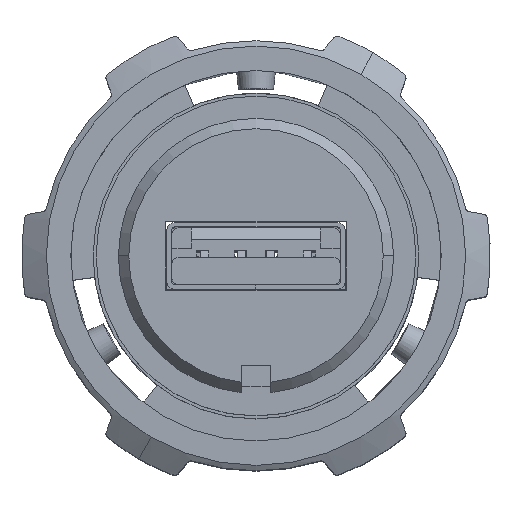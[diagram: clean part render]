
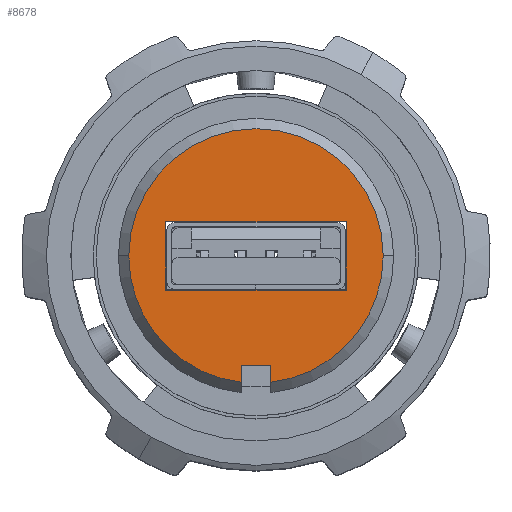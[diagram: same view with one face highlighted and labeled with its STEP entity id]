
A CAD part, top view. The second image highlights one B-rep face of the part: STEP entity #8678.
In plain terms, the highlighted face is planar.
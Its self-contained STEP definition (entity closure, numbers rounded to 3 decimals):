
#571 = ORIENTED_EDGE ( 'NONE', *, *, #32769, .F. ) ;
#1114 = VECTOR ( 'NONE', #8044, 1000. ) ;
#1284 = VERTEX_POINT ( 'NONE', #28945 ) ;
#1845 = ORIENTED_EDGE ( 'NONE', *, *, #14974, .F. ) ;
#2057 = DIRECTION ( 'NONE',  ( 0., 0., -1. ) ) ;
#2321 = LINE ( 'NONE', #23483, #1114 ) ;
#2483 = CIRCLE ( 'NONE', #13018, 8.55 ) ;
#3827 = EDGE_CURVE ( 'NONE', #29091, #33303, #2321, .T. ) ;
#4218 = DIRECTION ( 'NONE',  ( 0., -1., 0. ) ) ;
#4243 = ORIENTED_EDGE ( 'NONE', *, *, #15175, .F. ) ;
#4563 = LINE ( 'NONE', #15160, #25187 ) ;
#5226 = DIRECTION ( 'NONE',  ( 0., 0., -1. ) ) ;
#5228 = VERTEX_POINT ( 'NONE', #34061 ) ;
#5589 = VERTEX_POINT ( 'NONE', #20639 ) ;
#6197 = LINE ( 'NONE', #6367, #14381 ) ;
#6367 = CARTESIAN_POINT ( 'NONE',  ( -27.9, -2.3, 0. ) ) ;
#6452 = LINE ( 'NONE', #23599, #9389 ) ;
#6960 = VERTEX_POINT ( 'NONE', #18291 ) ;
#7272 = EDGE_LOOP ( 'NONE', ( #11603, #23255, #19505, #8201 ) ) ;
#7337 = FACE_OUTER_BOUND ( 'NONE', #19767, .T. ) ;
#7971 = AXIS2_PLACEMENT_3D ( 'NONE', #21669, #32272, #32097 ) ;
#8044 = DIRECTION ( 'NONE',  ( 0., -1., 0. ) ) ;
#8084 = VERTEX_POINT ( 'NONE', #21839 ) ;
#8201 = ORIENTED_EDGE ( 'NONE', *, *, #18964, .F. ) ;
#8480 = CARTESIAN_POINT ( 'NONE',  ( -27.9, -2.3, 6.05 ) ) ;
#8678 = ADVANCED_FACE ( 'NONE', ( #20852, #7337 ), #28850, .F. ) ;
#9386 = VECTOR ( 'NONE', #15297, 1000. ) ;
#9389 = VECTOR ( 'NONE', #17720, 1000. ) ;
#9442 = CARTESIAN_POINT ( 'NONE',  ( -27.9, 0., 8.55 ) ) ;
#9925 = LINE ( 'NONE', #15817, #9386 ) ;
#11046 = VECTOR ( 'NONE', #2057, 1000. ) ;
#11603 = ORIENTED_EDGE ( 'NONE', *, *, #29105, .F. ) ;
#12642 = CARTESIAN_POINT ( 'NONE',  ( -27.9, 2.3, 0. ) ) ;
#12925 = CIRCLE ( 'NONE', #32345, 8.55 ) ;
#13018 = AXIS2_PLACEMENT_3D ( 'NONE', #28632, #20814, #15802 ) ;
#14381 = VECTOR ( 'NONE', #32923, 1000. ) ;
#14974 = EDGE_CURVE ( 'NONE', #1284, #33925, #12925, .T. ) ;
#15160 = CARTESIAN_POINT ( 'NONE',  ( -27.9, 0., -1. ) ) ;
#15175 = EDGE_CURVE ( 'NONE', #5589, #1284, #26248, .T. ) ;
#15255 = LINE ( 'NONE', #12642, #11046 ) ;
#15297 = DIRECTION ( 'NONE',  ( 0., 1., 0. ) ) ;
#15527 = CARTESIAN_POINT ( 'NONE',  ( -27.9, -7.396, -1. ) ) ;
#15802 = DIRECTION ( 'NONE',  ( 0., 0., -1. ) ) ;
#15817 = CARTESIAN_POINT ( 'NONE',  ( -27.9, 0., 1. ) ) ;
#17163 = VECTOR ( 'NONE', #5226, 1000. ) ;
#17720 = DIRECTION ( 'NONE',  ( 0., 1., 0. ) ) ;
#17922 = DIRECTION ( 'NONE',  ( 0., 0., -1. ) ) ;
#18291 = CARTESIAN_POINT ( 'NONE',  ( -27.9, -8.491, 1. ) ) ;
#18566 = EDGE_CURVE ( 'NONE', #6960, #5228, #9925, .T. ) ;
#18964 = EDGE_CURVE ( 'NONE', #8084, #29091, #15255, .T. ) ;
#19505 = ORIENTED_EDGE ( 'NONE', *, *, #3827, .F. ) ;
#19623 = CARTESIAN_POINT ( 'NONE',  ( -27.9, 2.3, -6.05 ) ) ;
#19640 = CARTESIAN_POINT ( 'NONE',  ( -27.9, 0., 0. ) ) ;
#19767 = EDGE_LOOP ( 'NONE', ( #32640, #29613, #1845, #4243, #571, #33264 ) ) ;
#20324 = LINE ( 'NONE', #23262, #17163 ) ;
#20639 = CARTESIAN_POINT ( 'NONE',  ( -27.9, -8.491, -1. ) ) ;
#20650 = CARTESIAN_POINT ( 'NONE',  ( -27.9, -2.3, -6.05 ) ) ;
#20814 = DIRECTION ( 'NONE',  ( 1., 0., 0. ) ) ;
#20852 = FACE_BOUND ( 'NONE', #7272, .T. ) ;
#21669 = CARTESIAN_POINT ( 'NONE',  ( -27.9, 0., 0. ) ) ;
#21839 = CARTESIAN_POINT ( 'NONE',  ( -27.9, 2.3, 6.05 ) ) ;
#22414 = DIRECTION ( 'NONE',  ( 1., 0., 0. ) ) ;
#22799 = VERTEX_POINT ( 'NONE', #15527 ) ;
#23255 = ORIENTED_EDGE ( 'NONE', *, *, #27849, .F. ) ;
#23262 = CARTESIAN_POINT ( 'NONE',  ( -27.9, -7.396, 0. ) ) ;
#23483 = CARTESIAN_POINT ( 'NONE',  ( -27.9, 0., -6.05 ) ) ;
#23599 = CARTESIAN_POINT ( 'NONE',  ( -27.9, 0., 6.05 ) ) ;
#24695 = DIRECTION ( 'NONE',  ( 0., 0., -1. ) ) ;
#25187 = VECTOR ( 'NONE', #4218, 1000. ) ;
#25219 = VERTEX_POINT ( 'NONE', #8480 ) ;
#26248 = CIRCLE ( 'NONE', #7971, 8.55 ) ;
#27849 = EDGE_CURVE ( 'NONE', #33303, #25219, #6197, .T. ) ;
#28632 = CARTESIAN_POINT ( 'NONE',  ( -27.9, 0., 0. ) ) ;
#28850 = PLANE ( 'NONE',  #31919 ) ;
#28945 = CARTESIAN_POINT ( 'NONE',  ( -27.9, 0., -8.55 ) ) ;
#29091 = VERTEX_POINT ( 'NONE', #19623 ) ;
#29105 = EDGE_CURVE ( 'NONE', #25219, #8084, #6452, .T. ) ;
#29613 = ORIENTED_EDGE ( 'NONE', *, *, #33300, .F. ) ;
#29975 = EDGE_CURVE ( 'NONE', #5228, #22799, #20324, .T. ) ;
#31442 = DIRECTION ( 'NONE',  ( 1., 0., 0. ) ) ;
#31919 = AXIS2_PLACEMENT_3D ( 'NONE', #34071, #31442, #17922 ) ;
#32097 = DIRECTION ( 'NONE',  ( 0., 0., -1. ) ) ;
#32272 = DIRECTION ( 'NONE',  ( 1., 0., 0. ) ) ;
#32345 = AXIS2_PLACEMENT_3D ( 'NONE', #19640, #22414, #24695 ) ;
#32640 = ORIENTED_EDGE ( 'NONE', *, *, #18566, .F. ) ;
#32769 = EDGE_CURVE ( 'NONE', #22799, #5589, #4563, .T. ) ;
#32923 = DIRECTION ( 'NONE',  ( 0., 0., 1. ) ) ;
#33264 = ORIENTED_EDGE ( 'NONE', *, *, #29975, .F. ) ;
#33300 = EDGE_CURVE ( 'NONE', #33925, #6960, #2483, .T. ) ;
#33303 = VERTEX_POINT ( 'NONE', #20650 ) ;
#33925 = VERTEX_POINT ( 'NONE', #9442 ) ;
#34061 = CARTESIAN_POINT ( 'NONE',  ( -27.9, -7.396, 1. ) ) ;
#34071 = CARTESIAN_POINT ( 'NONE',  ( -27.9, 0., 0. ) ) ;
